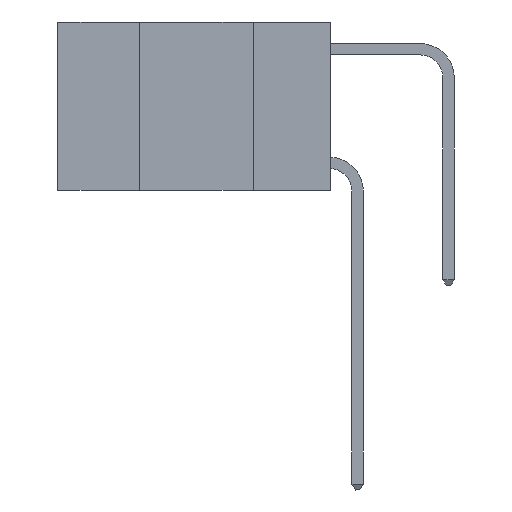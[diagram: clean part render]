
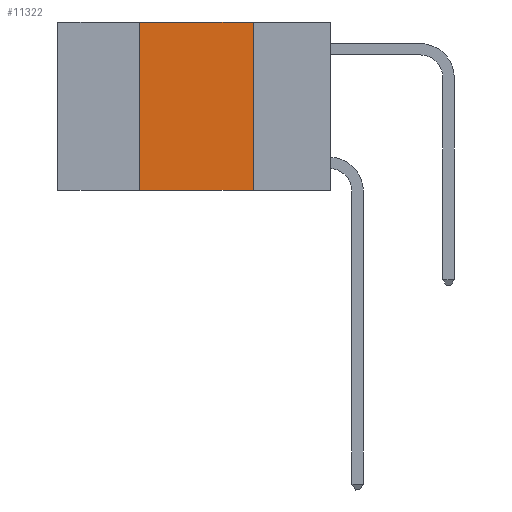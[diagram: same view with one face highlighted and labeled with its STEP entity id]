
A CAD part, left-side view. The second image highlights one B-rep face of the part: STEP entity #11322.
In plain terms, the highlighted planar face has unit normal (-1, 0, 0).
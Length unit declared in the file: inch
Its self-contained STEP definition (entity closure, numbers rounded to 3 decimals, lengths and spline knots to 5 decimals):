
#16 = ORIENTED_EDGE ( 'NONE', *, *, #10248, .F. ) ;
#279 = AXIS2_PLACEMENT_3D ( 'NONE', #7132, #9969, #5347 ) ;
#856 = VERTEX_POINT ( 'NONE', #7907 ) ;
#1267 = EDGE_LOOP ( 'NONE', ( #18230, #16, #13273, #18276 ) ) ;
#1676 = EDGE_CURVE ( 'NONE', #7208, #14731, #16767, .T. ) ;
#3817 = VECTOR ( 'NONE', #17298, 39.37008 ) ;
#4212 = CARTESIAN_POINT ( 'NONE',  ( 0., 0.42, 0. ) ) ;
#5347 = DIRECTION ( 'NONE',  ( 0., 0., -1. ) ) ;
#6732 = FACE_OUTER_BOUND ( 'NONE', #1267, .T. ) ;
#7132 = CARTESIAN_POINT ( 'NONE',  ( 0., 0.6, 0. ) ) ;
#7139 = VECTOR ( 'NONE', #18327, 39.37008 ) ;
#7208 = VERTEX_POINT ( 'NONE', #9033 ) ;
#7894 = EDGE_CURVE ( 'NONE', #856, #8990, #18976, .T. ) ;
#7907 = CARTESIAN_POINT ( 'NONE',  ( 0., 0.17, 0. ) ) ;
#7965 = DIRECTION ( 'NONE',  ( 0., -1., 0. ) ) ;
#8693 = CARTESIAN_POINT ( 'NONE',  ( 0., 0.42, 0. ) ) ;
#8990 = VERTEX_POINT ( 'NONE', #18169 ) ;
#9033 = CARTESIAN_POINT ( 'NONE',  ( 0., 0.42, -0.37 ) ) ;
#9969 = DIRECTION ( 'NONE',  ( 1., 0., 0. ) ) ;
#10179 = PLANE ( 'NONE',  #279 ) ;
#10248 = EDGE_CURVE ( 'NONE', #14731, #856, #19459, .T. ) ;
#11322 = ADVANCED_FACE ( 'NONE', ( #6732 ), #10179, .F. ) ;
#12681 = CARTESIAN_POINT ( 'NONE',  ( 0., 0.6, -0.37 ) ) ;
#12987 = CARTESIAN_POINT ( 'NONE',  ( 0., 0.17, 0. ) ) ;
#13273 = ORIENTED_EDGE ( 'NONE', *, *, #1676, .F. ) ;
#14102 = VECTOR ( 'NONE', #7965, 39.37008 ) ;
#14519 = DIRECTION ( 'NONE',  ( 0., -1., 0. ) ) ;
#14731 = VERTEX_POINT ( 'NONE', #4212 ) ;
#14732 = LINE ( 'NONE', #12681, #14102 ) ;
#15884 = CARTESIAN_POINT ( 'NONE',  ( 0., 0.6, 0. ) ) ;
#16336 = EDGE_CURVE ( 'NONE', #7208, #8990, #14732, .T. ) ;
#16767 = LINE ( 'NONE', #8693, #7139 ) ;
#17298 = DIRECTION ( 'NONE',  ( 0., 0., -1. ) ) ;
#18169 = CARTESIAN_POINT ( 'NONE',  ( 0., 0.17, -0.37 ) ) ;
#18230 = ORIENTED_EDGE ( 'NONE', *, *, #7894, .F. ) ;
#18276 = ORIENTED_EDGE ( 'NONE', *, *, #16336, .T. ) ;
#18327 = DIRECTION ( 'NONE',  ( 0., 0., 1. ) ) ;
#18976 = LINE ( 'NONE', #12987, #3817 ) ;
#19459 = LINE ( 'NONE', #15884, #20316 ) ;
#20316 = VECTOR ( 'NONE', #14519, 39.37008 ) ;
